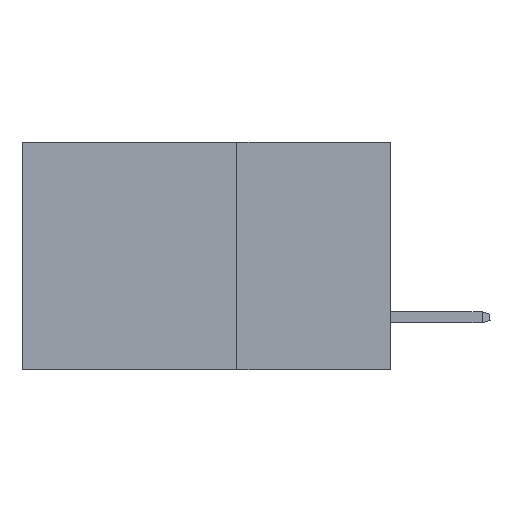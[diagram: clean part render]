
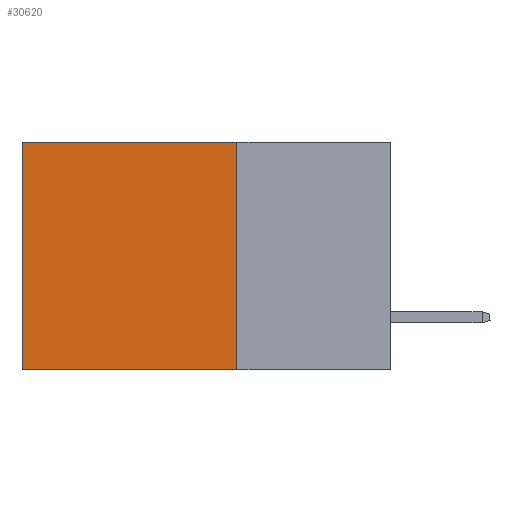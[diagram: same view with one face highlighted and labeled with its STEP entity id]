
A CAD part, left-side view. The second image highlights one B-rep face of the part: STEP entity #30620.
In plain terms, the highlighted planar face has unit normal (-1, 0, 0).
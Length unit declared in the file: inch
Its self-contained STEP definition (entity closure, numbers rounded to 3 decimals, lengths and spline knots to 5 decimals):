
#273 = CARTESIAN_POINT ( 'NONE',  ( 0.2875, 0.25, 0. ) ) ;
#1927 = CARTESIAN_POINT ( 'NONE',  ( 0.2875, 0.6, 0. ) ) ;
#3589 = ORIENTED_EDGE ( 'NONE', *, *, #31912, .F. ) ;
#3935 = DIRECTION ( 'NONE',  ( 0., 0., -1. ) ) ;
#5331 = DIRECTION ( 'NONE',  ( 0., 1., 0. ) ) ;
#6437 = VERTEX_POINT ( 'NONE', #26942 ) ;
#8230 = CARTESIAN_POINT ( 'NONE',  ( 0.2875, 0.25, 0. ) ) ;
#9226 = AXIS2_PLACEMENT_3D ( 'NONE', #16293, #20137, #16611 ) ;
#9501 = VECTOR ( 'NONE', #3935, 39.37008 ) ;
#10514 = VERTEX_POINT ( 'NONE', #8230 ) ;
#12812 = VECTOR ( 'NONE', #23067, 39.37008 ) ;
#12954 = PLANE ( 'NONE',  #9226 ) ;
#16293 = CARTESIAN_POINT ( 'NONE',  ( 0.2875, 0.25, 0. ) ) ;
#16611 = DIRECTION ( 'NONE',  ( 0., 0., -1. ) ) ;
#18974 = EDGE_CURVE ( 'NONE', #10514, #6437, #35285, .T. ) ;
#19875 = ORIENTED_EDGE ( 'NONE', *, *, #18974, .F. ) ;
#19917 = ORIENTED_EDGE ( 'NONE', *, *, #32570, .T. ) ;
#20137 = DIRECTION ( 'NONE',  ( 1., 0., 0. ) ) ;
#20662 = VECTOR ( 'NONE', #5331, 39.37008 ) ;
#21041 = CARTESIAN_POINT ( 'NONE',  ( 0.2875, 0.25, -0.37 ) ) ;
#21754 = LINE ( 'NONE', #1927, #48702 ) ;
#22981 = LINE ( 'NONE', #46523, #12812 ) ;
#23067 = DIRECTION ( 'NONE',  ( 0., 1., 0. ) ) ;
#23413 = FACE_OUTER_BOUND ( 'NONE', #29995, .T. ) ;
#24025 = VERTEX_POINT ( 'NONE', #33592 ) ;
#25144 = DIRECTION ( 'NONE',  ( 0., 0., -1. ) ) ;
#25702 = CARTESIAN_POINT ( 'NONE',  ( 0.2875, 0.6, -0.37 ) ) ;
#26942 = CARTESIAN_POINT ( 'NONE',  ( 0.2875, 0.25, -0.37 ) ) ;
#27821 = VERTEX_POINT ( 'NONE', #25702 ) ;
#29995 = EDGE_LOOP ( 'NONE', ( #19917, #3589, #19875, #32821 ) ) ;
#30620 = ADVANCED_FACE ( 'NONE', ( #23413 ), #12954, .F. ) ;
#31912 = EDGE_CURVE ( 'NONE', #6437, #27821, #45279, .T. ) ;
#32570 = EDGE_CURVE ( 'NONE', #24025, #27821, #21754, .T. ) ;
#32821 = ORIENTED_EDGE ( 'NONE', *, *, #44772, .T. ) ;
#33592 = CARTESIAN_POINT ( 'NONE',  ( 0.2875, 0.6, 0. ) ) ;
#35285 = LINE ( 'NONE', #273, #9501 ) ;
#44772 = EDGE_CURVE ( 'NONE', #10514, #24025, #22981, .T. ) ;
#45279 = LINE ( 'NONE', #21041, #20662 ) ;
#46523 = CARTESIAN_POINT ( 'NONE',  ( 0.2875, 0.25, 0. ) ) ;
#48702 = VECTOR ( 'NONE', #25144, 39.37008 ) ;
